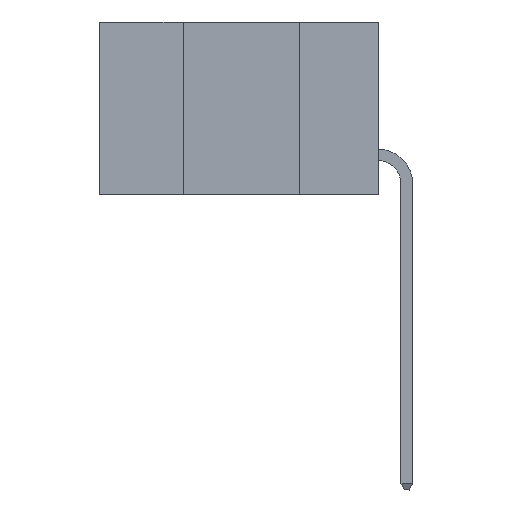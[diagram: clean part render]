
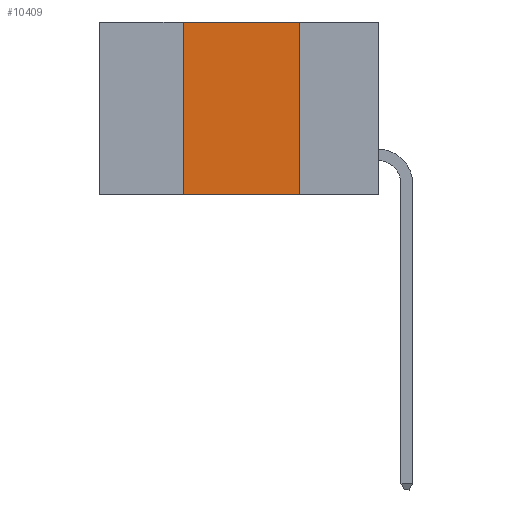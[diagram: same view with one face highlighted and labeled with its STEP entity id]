
A CAD part, left-side view. The second image highlights one B-rep face of the part: STEP entity #10409.
In plain terms, the highlighted planar face has unit normal (-1, 0, 0).
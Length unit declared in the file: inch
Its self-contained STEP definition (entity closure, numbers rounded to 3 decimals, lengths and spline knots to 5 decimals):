
#287 = DIRECTION ( 'NONE',  ( 0., -1., 0. ) ) ;
#1266 = ORIENTED_EDGE ( 'NONE', *, *, #17785, .F. ) ;
#1303 = VECTOR ( 'NONE', #9143, 39.37008 ) ;
#1331 = VECTOR ( 'NONE', #16481, 39.37008 ) ;
#1955 = CARTESIAN_POINT ( 'NONE',  ( 0., 0.6, -0.37 ) ) ;
#2363 = VERTEX_POINT ( 'NONE', #14518 ) ;
#3452 = EDGE_CURVE ( 'NONE', #18772, #4305, #14057, .T. ) ;
#4305 = VERTEX_POINT ( 'NONE', #21349 ) ;
#6339 = DIRECTION ( 'NONE',  ( 0., 0., -1. ) ) ;
#6631 = DIRECTION ( 'NONE',  ( 1., 0., 0. ) ) ;
#6645 = FACE_OUTER_BOUND ( 'NONE', #18858, .T. ) ;
#6768 = PLANE ( 'NONE',  #20340 ) ;
#7713 = VECTOR ( 'NONE', #287, 39.37008 ) ;
#7795 = ORIENTED_EDGE ( 'NONE', *, *, #19793, .F. ) ;
#9143 = DIRECTION ( 'NONE',  ( 0., 0., 1. ) ) ;
#9247 = CARTESIAN_POINT ( 'NONE',  ( 0., 0.6, 0. ) ) ;
#10409 = ADVANCED_FACE ( 'NONE', ( #6645 ), #6768, .F. ) ;
#12879 = CARTESIAN_POINT ( 'NONE',  ( 0., 0.42, 0. ) ) ;
#14057 = LINE ( 'NONE', #16714, #1331 ) ;
#14100 = CARTESIAN_POINT ( 'NONE',  ( 0., 0.17, -0.37 ) ) ;
#14518 = CARTESIAN_POINT ( 'NONE',  ( 0., 0.42, -0.37 ) ) ;
#15751 = LINE ( 'NONE', #17077, #19713 ) ;
#15821 = ORIENTED_EDGE ( 'NONE', *, *, #3452, .F. ) ;
#16481 = DIRECTION ( 'NONE',  ( 0., -1., 0. ) ) ;
#16714 = CARTESIAN_POINT ( 'NONE',  ( 0., 0.6, 0. ) ) ;
#17077 = CARTESIAN_POINT ( 'NONE',  ( 0., 0.17, 0. ) ) ;
#17164 = DIRECTION ( 'NONE',  ( 0., 0., -1. ) ) ;
#17785 = EDGE_CURVE ( 'NONE', #4305, #19788, #15751, .T. ) ;
#17970 = LINE ( 'NONE', #20815, #1303 ) ;
#18392 = EDGE_CURVE ( 'NONE', #2363, #19788, #20946, .T. ) ;
#18772 = VERTEX_POINT ( 'NONE', #12879 ) ;
#18858 = EDGE_LOOP ( 'NONE', ( #1266, #15821, #7795, #21604 ) ) ;
#19713 = VECTOR ( 'NONE', #17164, 39.37008 ) ;
#19788 = VERTEX_POINT ( 'NONE', #14100 ) ;
#19793 = EDGE_CURVE ( 'NONE', #2363, #18772, #17970, .T. ) ;
#20340 = AXIS2_PLACEMENT_3D ( 'NONE', #9247, #6631, #6339 ) ;
#20815 = CARTESIAN_POINT ( 'NONE',  ( 0., 0.42, 0. ) ) ;
#20946 = LINE ( 'NONE', #1955, #7713 ) ;
#21349 = CARTESIAN_POINT ( 'NONE',  ( 0., 0.17, 0. ) ) ;
#21604 = ORIENTED_EDGE ( 'NONE', *, *, #18392, .T. ) ;
